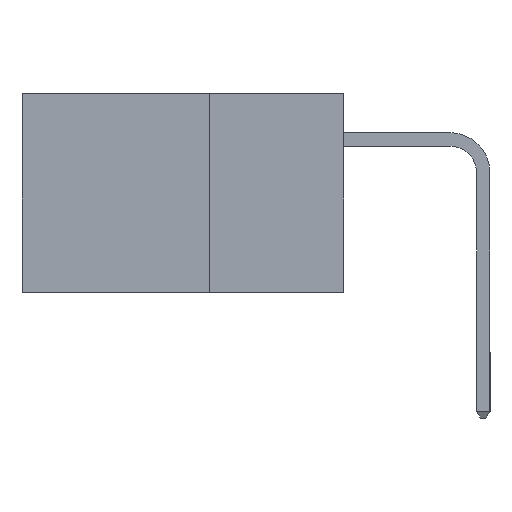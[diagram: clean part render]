
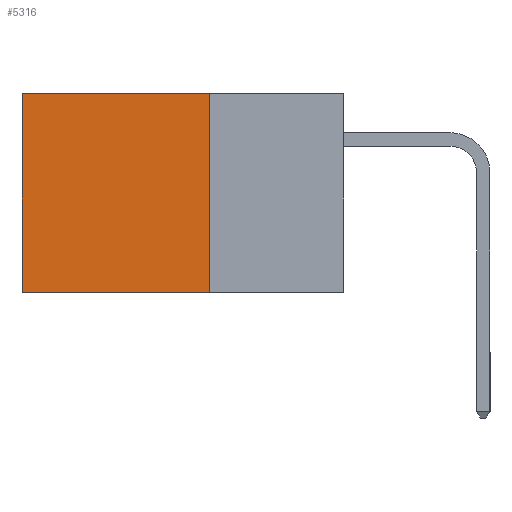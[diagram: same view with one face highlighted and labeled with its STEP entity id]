
A CAD part, left-side view. The second image highlights one B-rep face of the part: STEP entity #5316.
In plain terms, the highlighted planar face has unit normal (-1, 0, 0).
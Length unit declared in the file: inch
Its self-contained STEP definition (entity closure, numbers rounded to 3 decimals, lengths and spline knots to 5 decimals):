
#1174 = PLANE ( 'NONE',  #14358 ) ;
#1274 = DIRECTION ( 'NONE',  ( 1., 0., 0. ) ) ;
#1687 = VERTEX_POINT ( 'NONE', #17238 ) ;
#2194 = VERTEX_POINT ( 'NONE', #16114 ) ;
#2291 = EDGE_CURVE ( 'NONE', #2194, #5781, #15369, .T. ) ;
#2753 = VERTEX_POINT ( 'NONE', #15253 ) ;
#2852 = CARTESIAN_POINT ( 'NONE',  ( 0.2615, 0.6, -0.37 ) ) ;
#3679 = DIRECTION ( 'NONE',  ( 0., 0., -1. ) ) ;
#4224 = DIRECTION ( 'NONE',  ( 0., 0., -1. ) ) ;
#4749 = VECTOR ( 'NONE', #16915, 39.37008 ) ;
#5309 = DIRECTION ( 'NONE',  ( 0., 1., 0. ) ) ;
#5316 = ADVANCED_FACE ( 'NONE', ( #8266 ), #1174, .F. ) ;
#5338 = EDGE_CURVE ( 'NONE', #1687, #5781, #15378, .T. ) ;
#5781 = VERTEX_POINT ( 'NONE', #16179 ) ;
#5867 = CARTESIAN_POINT ( 'NONE',  ( 0.2615, 0.25, -0.37 ) ) ;
#5987 = EDGE_CURVE ( 'NONE', #2753, #2194, #16545, .T. ) ;
#6327 = ORIENTED_EDGE ( 'NONE', *, *, #5338, .T. ) ;
#6968 = LINE ( 'NONE', #15370, #15676 ) ;
#8266 = FACE_OUTER_BOUND ( 'NONE', #16912, .T. ) ;
#8268 = VECTOR ( 'NONE', #8435, 39.37008 ) ;
#8435 = DIRECTION ( 'NONE',  ( 0., 0., -1. ) ) ;
#9298 = ORIENTED_EDGE ( 'NONE', *, *, #12942, .T. ) ;
#12047 = ORIENTED_EDGE ( 'NONE', *, *, #2291, .F. ) ;
#12365 = CARTESIAN_POINT ( 'NONE',  ( 0.2615, 0.25, -0.37 ) ) ;
#12942 = EDGE_CURVE ( 'NONE', #2753, #1687, #6968, .T. ) ;
#14358 = AXIS2_PLACEMENT_3D ( 'NONE', #16560, #1274, #4224 ) ;
#14631 = VECTOR ( 'NONE', #3679, 39.37008 ) ;
#15253 = CARTESIAN_POINT ( 'NONE',  ( 0.2615, 0.25, 0. ) ) ;
#15369 = LINE ( 'NONE', #5867, #4749 ) ;
#15370 = CARTESIAN_POINT ( 'NONE',  ( 0.2615, 0.25, 0. ) ) ;
#15378 = LINE ( 'NONE', #2852, #14631 ) ;
#15676 = VECTOR ( 'NONE', #5309, 39.37008 ) ;
#15966 = ORIENTED_EDGE ( 'NONE', *, *, #5987, .F. ) ;
#16114 = CARTESIAN_POINT ( 'NONE',  ( 0.2615, 0.25, -0.37 ) ) ;
#16179 = CARTESIAN_POINT ( 'NONE',  ( 0.2615, 0.6, -0.37 ) ) ;
#16545 = LINE ( 'NONE', #12365, #8268 ) ;
#16560 = CARTESIAN_POINT ( 'NONE',  ( 0.2615, 0.25, -0.37 ) ) ;
#16912 = EDGE_LOOP ( 'NONE', ( #6327, #12047, #15966, #9298 ) ) ;
#16915 = DIRECTION ( 'NONE',  ( 0., 1., 0. ) ) ;
#17238 = CARTESIAN_POINT ( 'NONE',  ( 0.2615, 0.6, 0. ) ) ;
